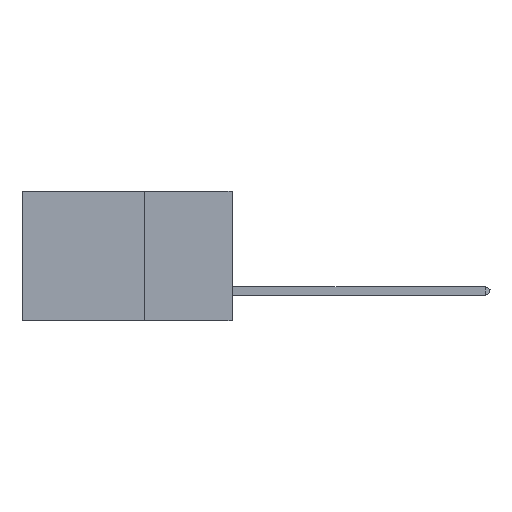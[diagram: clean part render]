
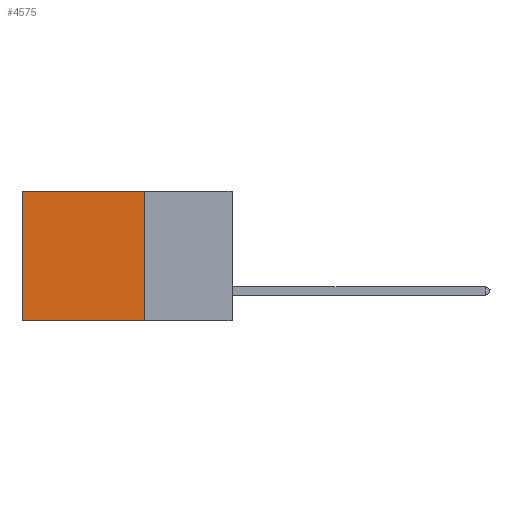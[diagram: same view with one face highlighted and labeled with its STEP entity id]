
A CAD part, left-side view. The second image highlights one B-rep face of the part: STEP entity #4575.
In plain terms, the highlighted planar face has unit normal (-1, 0, 0).
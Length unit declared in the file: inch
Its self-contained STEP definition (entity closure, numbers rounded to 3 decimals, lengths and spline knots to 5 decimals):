
#260 = ORIENTED_EDGE ( 'NONE', *, *, #15857, .T. ) ;
#440 = DIRECTION ( 'NONE',  ( 0., 0., -1. ) ) ;
#3417 = AXIS2_PLACEMENT_3D ( 'NONE', #14643, #9686, #17221 ) ;
#4575 = ADVANCED_FACE ( 'NONE', ( #25107 ), #32430, .F. ) ;
#5677 = CARTESIAN_POINT ( 'NONE',  ( 0.2875, 0.25, 0. ) ) ;
#6355 = VERTEX_POINT ( 'NONE', #15865 ) ;
#7891 = CARTESIAN_POINT ( 'NONE',  ( 0.2875, 0.6, 0. ) ) ;
#8834 = CARTESIAN_POINT ( 'NONE',  ( 0.2875, 0.25, -0.37 ) ) ;
#9196 = CARTESIAN_POINT ( 'NONE',  ( 0.2875, 0.25, -0.37 ) ) ;
#9686 = DIRECTION ( 'NONE',  ( 1., 0., 0. ) ) ;
#9864 = VECTOR ( 'NONE', #11989, 39.37008 ) ;
#9878 = VERTEX_POINT ( 'NONE', #8834 ) ;
#11989 = DIRECTION ( 'NONE',  ( 0., 1., 0. ) ) ;
#12104 = DIRECTION ( 'NONE',  ( 0., 1., 0. ) ) ;
#12512 = VERTEX_POINT ( 'NONE', #27787 ) ;
#12863 = VERTEX_POINT ( 'NONE', #14997 ) ;
#14272 = LINE ( 'NONE', #27488, #9864 ) ;
#14377 = EDGE_CURVE ( 'NONE', #12863, #9878, #24831, .T. ) ;
#14643 = CARTESIAN_POINT ( 'NONE',  ( 0.2875, 0.25, 0. ) ) ;
#14997 = CARTESIAN_POINT ( 'NONE',  ( 0.2875, 0.25, 0. ) ) ;
#15379 = ORIENTED_EDGE ( 'NONE', *, *, #27797, .F. ) ;
#15857 = EDGE_CURVE ( 'NONE', #6355, #12512, #30697, .T. ) ;
#15865 = CARTESIAN_POINT ( 'NONE',  ( 0.2875, 0.6, 0. ) ) ;
#17221 = DIRECTION ( 'NONE',  ( 0., 0., -1. ) ) ;
#20656 = ORIENTED_EDGE ( 'NONE', *, *, #14377, .F. ) ;
#21105 = DIRECTION ( 'NONE',  ( 0., 0., -1. ) ) ;
#21471 = EDGE_CURVE ( 'NONE', #12863, #6355, #14272, .T. ) ;
#23142 = LINE ( 'NONE', #9196, #32332 ) ;
#24725 = ORIENTED_EDGE ( 'NONE', *, *, #21471, .T. ) ;
#24831 = LINE ( 'NONE', #5677, #27628 ) ;
#25107 = FACE_OUTER_BOUND ( 'NONE', #28061, .T. ) ;
#26705 = VECTOR ( 'NONE', #440, 39.37008 ) ;
#27488 = CARTESIAN_POINT ( 'NONE',  ( 0.2875, 0.25, 0. ) ) ;
#27628 = VECTOR ( 'NONE', #21105, 39.37008 ) ;
#27787 = CARTESIAN_POINT ( 'NONE',  ( 0.2875, 0.6, -0.37 ) ) ;
#27797 = EDGE_CURVE ( 'NONE', #9878, #12512, #23142, .T. ) ;
#28061 = EDGE_LOOP ( 'NONE', ( #260, #15379, #20656, #24725 ) ) ;
#30697 = LINE ( 'NONE', #7891, #26705 ) ;
#32332 = VECTOR ( 'NONE', #12104, 39.37008 ) ;
#32430 = PLANE ( 'NONE',  #3417 ) ;
